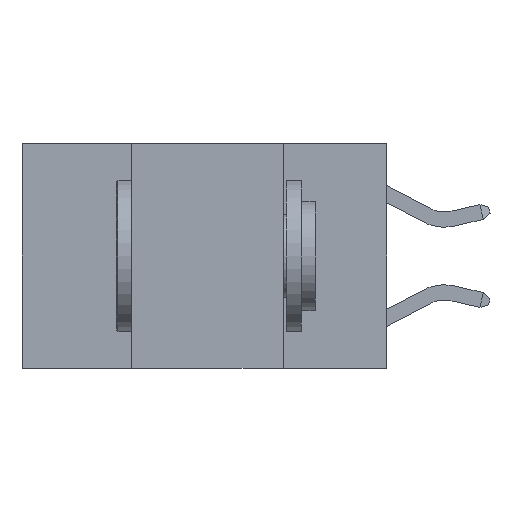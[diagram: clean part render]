
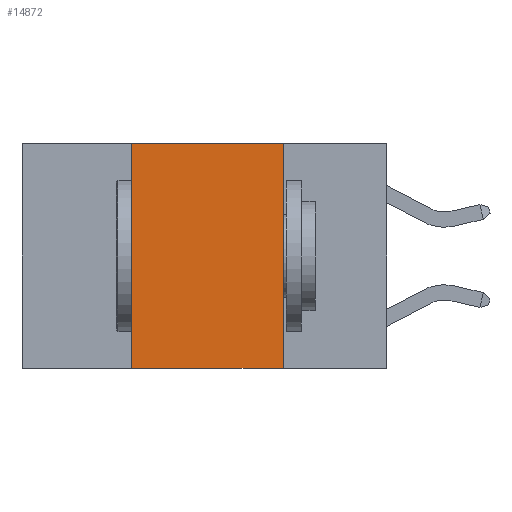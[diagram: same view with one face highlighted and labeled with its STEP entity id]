
A CAD part, left-side view. The second image highlights one B-rep face of the part: STEP entity #14872.
In plain terms, the highlighted planar face has unit normal (-1, 0, 0).
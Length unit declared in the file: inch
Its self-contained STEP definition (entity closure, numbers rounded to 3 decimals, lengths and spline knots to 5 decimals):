
#846 = CARTESIAN_POINT ( 'NONE',  ( 0., 0.17, 0. ) ) ;
#1240 = VECTOR ( 'NONE', #2161, 39.37008 ) ;
#1530 = AXIS2_PLACEMENT_3D ( 'NONE', #13858, #4688, #15371 ) ;
#2161 = DIRECTION ( 'NONE',  ( 0., -1., 0. ) ) ;
#2196 = ORIENTED_EDGE ( 'NONE', *, *, #2330, .F. ) ;
#2278 = DIRECTION ( 'NONE',  ( 0., 0., -1. ) ) ;
#2330 = EDGE_CURVE ( 'NONE', #9482, #7334, #8038, .T. ) ;
#2601 = VECTOR ( 'NONE', #19326, 39.37008 ) ;
#3089 = LINE ( 'NONE', #17833, #2601 ) ;
#3178 = PLANE ( 'NONE',  #1530 ) ;
#4688 = DIRECTION ( 'NONE',  ( 1., 0., 0. ) ) ;
#6221 = VERTEX_POINT ( 'NONE', #19066 ) ;
#7334 = VERTEX_POINT ( 'NONE', #14223 ) ;
#7526 = CARTESIAN_POINT ( 'NONE',  ( 0., 0.6, -0.37 ) ) ;
#7863 = LINE ( 'NONE', #7526, #15487 ) ;
#8038 = LINE ( 'NONE', #846, #15181 ) ;
#8490 = FACE_OUTER_BOUND ( 'NONE', #13614, .T. ) ;
#8840 = LINE ( 'NONE', #9745, #1240 ) ;
#9052 = DIRECTION ( 'NONE',  ( 0., -1., 0. ) ) ;
#9482 = VERTEX_POINT ( 'NONE', #9651 ) ;
#9590 = CARTESIAN_POINT ( 'NONE',  ( 0., 0.42, -0.37 ) ) ;
#9651 = CARTESIAN_POINT ( 'NONE',  ( 0., 0.17, 0. ) ) ;
#9745 = CARTESIAN_POINT ( 'NONE',  ( 0., 0.6, 0. ) ) ;
#12357 = EDGE_CURVE ( 'NONE', #6221, #9482, #8840, .T. ) ;
#13166 = EDGE_CURVE ( 'NONE', #16358, #6221, #3089, .T. ) ;
#13326 = EDGE_CURVE ( 'NONE', #16358, #7334, #7863, .T. ) ;
#13614 = EDGE_LOOP ( 'NONE', ( #2196, #18619, #17302, #17730 ) ) ;
#13858 = CARTESIAN_POINT ( 'NONE',  ( 0., 0.6, 0. ) ) ;
#14223 = CARTESIAN_POINT ( 'NONE',  ( 0., 0.17, -0.37 ) ) ;
#14872 = ADVANCED_FACE ( 'NONE', ( #8490 ), #3178, .F. ) ;
#15181 = VECTOR ( 'NONE', #2278, 39.37008 ) ;
#15371 = DIRECTION ( 'NONE',  ( 0., 0., -1. ) ) ;
#15487 = VECTOR ( 'NONE', #9052, 39.37008 ) ;
#16358 = VERTEX_POINT ( 'NONE', #9590 ) ;
#17302 = ORIENTED_EDGE ( 'NONE', *, *, #13166, .F. ) ;
#17730 = ORIENTED_EDGE ( 'NONE', *, *, #13326, .T. ) ;
#17833 = CARTESIAN_POINT ( 'NONE',  ( 0., 0.42, 0. ) ) ;
#18619 = ORIENTED_EDGE ( 'NONE', *, *, #12357, .F. ) ;
#19066 = CARTESIAN_POINT ( 'NONE',  ( 0., 0.42, 0. ) ) ;
#19326 = DIRECTION ( 'NONE',  ( 0., 0., 1. ) ) ;
